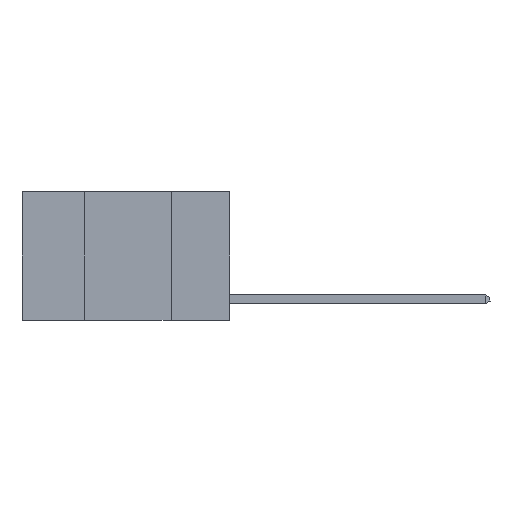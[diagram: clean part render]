
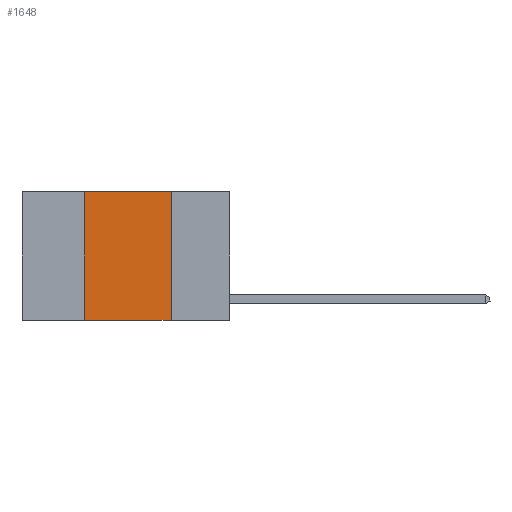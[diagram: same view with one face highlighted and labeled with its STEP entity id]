
A CAD part, left-side view. The second image highlights one B-rep face of the part: STEP entity #1648.
In plain terms, the highlighted planar face has unit normal (-1, 0, 0).
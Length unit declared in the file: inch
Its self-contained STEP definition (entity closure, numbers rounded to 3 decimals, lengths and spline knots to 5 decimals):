
#279 = LINE ( 'NONE', #5009, #2949 ) ;
#1487 = LINE ( 'NONE', #14586, #16508 ) ;
#1648 = ADVANCED_FACE ( 'NONE', ( #10166 ), #12327, .F. ) ;
#2664 = AXIS2_PLACEMENT_3D ( 'NONE', #12133, #12117, #12061 ) ;
#2949 = VECTOR ( 'NONE', #6611, 39.37008 ) ;
#3923 = VECTOR ( 'NONE', #15755, 39.37008 ) ;
#4701 = VERTEX_POINT ( 'NONE', #9692 ) ;
#5009 = CARTESIAN_POINT ( 'NONE',  ( 0., 0.17, 0. ) ) ;
#5146 = CARTESIAN_POINT ( 'NONE',  ( 0., 0.6, -0.37 ) ) ;
#6234 = VERTEX_POINT ( 'NONE', #18119 ) ;
#6525 = EDGE_CURVE ( 'NONE', #4701, #6234, #19741, .T. ) ;
#6561 = EDGE_CURVE ( 'NONE', #12416, #7547, #279, .T. ) ;
#6611 = DIRECTION ( 'NONE',  ( 0., 0., -1. ) ) ;
#6623 = EDGE_CURVE ( 'NONE', #4701, #7547, #14371, .T. ) ;
#7547 = VERTEX_POINT ( 'NONE', #15473 ) ;
#7707 = EDGE_LOOP ( 'NONE', ( #11120, #11593, #15673, #12077 ) ) ;
#9612 = CARTESIAN_POINT ( 'NONE',  ( 0., 0.42, 0. ) ) ;
#9692 = CARTESIAN_POINT ( 'NONE',  ( 0., 0.42, -0.37 ) ) ;
#10166 = FACE_OUTER_BOUND ( 'NONE', #7707, .T. ) ;
#11120 = ORIENTED_EDGE ( 'NONE', *, *, #6561, .F. ) ;
#11593 = ORIENTED_EDGE ( 'NONE', *, *, #17819, .F. ) ;
#12061 = DIRECTION ( 'NONE',  ( 0., 0., -1. ) ) ;
#12077 = ORIENTED_EDGE ( 'NONE', *, *, #6623, .T. ) ;
#12117 = DIRECTION ( 'NONE',  ( 1., 0., 0. ) ) ;
#12133 = CARTESIAN_POINT ( 'NONE',  ( 0., 0.6, 0. ) ) ;
#12327 = PLANE ( 'NONE',  #2664 ) ;
#12416 = VERTEX_POINT ( 'NONE', #12788 ) ;
#12788 = CARTESIAN_POINT ( 'NONE',  ( 0., 0.17, 0. ) ) ;
#14371 = LINE ( 'NONE', #5146, #14858 ) ;
#14586 = CARTESIAN_POINT ( 'NONE',  ( 0., 0.6, 0. ) ) ;
#14858 = VECTOR ( 'NONE', #17514, 39.37008 ) ;
#15473 = CARTESIAN_POINT ( 'NONE',  ( 0., 0.17, -0.37 ) ) ;
#15673 = ORIENTED_EDGE ( 'NONE', *, *, #6525, .F. ) ;
#15755 = DIRECTION ( 'NONE',  ( 0., 0., 1. ) ) ;
#16101 = DIRECTION ( 'NONE',  ( 0., -1., 0. ) ) ;
#16508 = VECTOR ( 'NONE', #16101, 39.37008 ) ;
#17514 = DIRECTION ( 'NONE',  ( 0., -1., 0. ) ) ;
#17819 = EDGE_CURVE ( 'NONE', #6234, #12416, #1487, .T. ) ;
#18119 = CARTESIAN_POINT ( 'NONE',  ( 0., 0.42, 0. ) ) ;
#19741 = LINE ( 'NONE', #9612, #3923 ) ;
